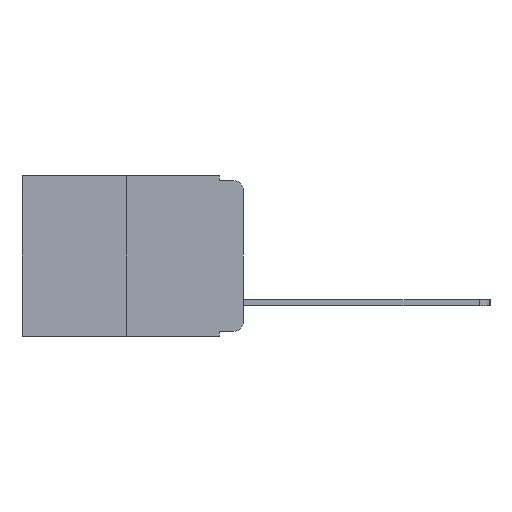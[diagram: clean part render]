
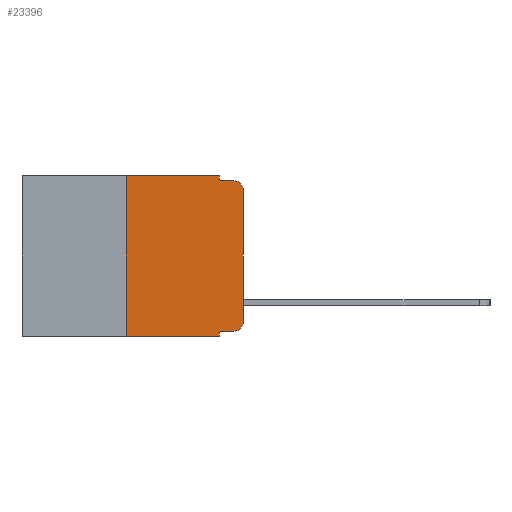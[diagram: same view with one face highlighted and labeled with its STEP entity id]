
A CAD part, left-side view. The second image highlights one B-rep face of the part: STEP entity #23396.
In plain terms, the highlighted planar face has unit normal (-1, 0, 0).
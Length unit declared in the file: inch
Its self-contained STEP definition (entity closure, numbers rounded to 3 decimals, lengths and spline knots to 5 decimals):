
#172 = LINE ( 'NONE', #19578, #9932 ) ;
#1285 = VERTEX_POINT ( 'NONE', #12604 ) ;
#1417 = ORIENTED_EDGE ( 'NONE', *, *, #24601, .T. ) ;
#1732 = CARTESIAN_POINT ( 'NONE',  ( 0., 0., -0.03 ) ) ;
#2103 = CARTESIAN_POINT ( 'NONE',  ( 0., 0.473, 0. ) ) ;
#2247 = FACE_OUTER_BOUND ( 'NONE', #20604, .T. ) ;
#2303 = CARTESIAN_POINT ( 'NONE',  ( 0., 0., 0. ) ) ;
#2648 = VERTEX_POINT ( 'NONE', #5030 ) ;
#3129 = CARTESIAN_POINT ( 'NONE',  ( 0., 0.051, -0.01 ) ) ;
#3479 = CARTESIAN_POINT ( 'NONE',  ( 0., 0.02, -0.333 ) ) ;
#3543 = ORIENTED_EDGE ( 'NONE', *, *, #11401, .T. ) ;
#3576 = VECTOR ( 'NONE', #8327, 39.37008 ) ;
#3725 = VERTEX_POINT ( 'NONE', #11868 ) ;
#3742 = EDGE_CURVE ( 'NONE', #19239, #2648, #11550, .T. ) ;
#4079 = DIRECTION ( 'NONE',  ( 0., 0., -1. ) ) ;
#4282 = DIRECTION ( 'NONE',  ( 0., 0., 1. ) ) ;
#4989 = CARTESIAN_POINT ( 'NONE',  ( 0., 0.25, 0. ) ) ;
#5030 = CARTESIAN_POINT ( 'NONE',  ( 0., 0., -0.313 ) ) ;
#5317 = VERTEX_POINT ( 'NONE', #4989 ) ;
#5421 = CARTESIAN_POINT ( 'NONE',  ( 0., 0.051, -0.01 ) ) ;
#5952 = VECTOR ( 'NONE', #24558, 39.37008 ) ;
#5959 = VECTOR ( 'NONE', #7325, 39.37008 ) ;
#6281 = CIRCLE ( 'NONE', #14288, 0.02 ) ;
#6355 = ORIENTED_EDGE ( 'NONE', *, *, #17832, .F. ) ;
#6842 = VERTEX_POINT ( 'NONE', #1732 ) ;
#7205 = EDGE_CURVE ( 'NONE', #6842, #19594, #6281, .T. ) ;
#7266 = ORIENTED_EDGE ( 'NONE', *, *, #7205, .T. ) ;
#7325 = DIRECTION ( 'NONE',  ( 0., -1., 0. ) ) ;
#7540 = VECTOR ( 'NONE', #11343, 39.37008 ) ;
#8327 = DIRECTION ( 'NONE',  ( 0., -1., 0. ) ) ;
#8449 = CARTESIAN_POINT ( 'NONE',  ( 0., 0.473, 0. ) ) ;
#8485 = ORIENTED_EDGE ( 'NONE', *, *, #20113, .F. ) ;
#8624 = CARTESIAN_POINT ( 'NONE',  ( 0., 0.02, -0.01 ) ) ;
#8637 = VECTOR ( 'NONE', #4282, 39.37008 ) ;
#9074 = ORIENTED_EDGE ( 'NONE', *, *, #22589, .F. ) ;
#9227 = LINE ( 'NONE', #2303, #8637 ) ;
#9397 = CARTESIAN_POINT ( 'NONE',  ( 0., 0.051, 0. ) ) ;
#9544 = VERTEX_POINT ( 'NONE', #23968 ) ;
#9932 = VECTOR ( 'NONE', #23350, 39.37008 ) ;
#10011 = CARTESIAN_POINT ( 'NONE',  ( 0., 0.02, -0.313 ) ) ;
#10608 = CARTESIAN_POINT ( 'NONE',  ( 0., 0.02, -0.03 ) ) ;
#11343 = DIRECTION ( 'NONE',  ( 0., 0., -1. ) ) ;
#11401 = EDGE_CURVE ( 'NONE', #13711, #19239, #13958, .T. ) ;
#11477 = ORIENTED_EDGE ( 'NONE', *, *, #22832, .F. ) ;
#11550 = CIRCLE ( 'NONE', #17213, 0.02 ) ;
#11707 = LINE ( 'NONE', #15319, #5952 ) ;
#11868 = CARTESIAN_POINT ( 'NONE',  ( 0., 0.051, 0. ) ) ;
#11964 = DIRECTION ( 'NONE',  ( 0., 0., -1. ) ) ;
#12585 = DIRECTION ( 'NONE',  ( 0., 0., -1. ) ) ;
#12604 = CARTESIAN_POINT ( 'NONE',  ( 0., 0.051, -0.343 ) ) ;
#12703 = LINE ( 'NONE', #9397, #7540 ) ;
#13164 = VECTOR ( 'NONE', #22785, 39.37008 ) ;
#13711 = VERTEX_POINT ( 'NONE', #20952 ) ;
#13756 = LINE ( 'NONE', #20962, #13164 ) ;
#13958 = LINE ( 'NONE', #16002, #3576 ) ;
#14231 = EDGE_CURVE ( 'NONE', #9544, #1285, #11707, .T. ) ;
#14288 = AXIS2_PLACEMENT_3D ( 'NONE', #10608, #23798, #12585 ) ;
#15319 = CARTESIAN_POINT ( 'NONE',  ( 0., 0.473, -0.343 ) ) ;
#15429 = ORIENTED_EDGE ( 'NONE', *, *, #21897, .F. ) ;
#15718 = DIRECTION ( 'NONE',  ( 1., 0., 0. ) ) ;
#16002 = CARTESIAN_POINT ( 'NONE',  ( 0., 0.051, -0.333 ) ) ;
#16252 = LINE ( 'NONE', #5421, #5959 ) ;
#17094 = LINE ( 'NONE', #8449, #22614 ) ;
#17213 = AXIS2_PLACEMENT_3D ( 'NONE', #10011, #23212, #11964 ) ;
#17832 = EDGE_CURVE ( 'NONE', #5317, #3725, #17094, .T. ) ;
#19239 = VERTEX_POINT ( 'NONE', #3479 ) ;
#19391 = PLANE ( 'NONE',  #20405 ) ;
#19526 = ORIENTED_EDGE ( 'NONE', *, *, #3742, .T. ) ;
#19578 = CARTESIAN_POINT ( 'NONE',  ( 0., 0.25, 0. ) ) ;
#19594 = VERTEX_POINT ( 'NONE', #8624 ) ;
#19877 = DIRECTION ( 'NONE',  ( 0., -1., 0. ) ) ;
#20113 = EDGE_CURVE ( 'NONE', #13711, #1285, #13756, .T. ) ;
#20405 = AXIS2_PLACEMENT_3D ( 'NONE', #2103, #15718, #4079 ) ;
#20602 = VERTEX_POINT ( 'NONE', #3129 ) ;
#20604 = EDGE_LOOP ( 'NONE', ( #1417, #7266, #9074, #15429, #6355, #11477, #22133, #8485, #3543, #19526 ) ) ;
#20952 = CARTESIAN_POINT ( 'NONE',  ( 0., 0.051, -0.333 ) ) ;
#20962 = CARTESIAN_POINT ( 'NONE',  ( 0., 0.051, 0. ) ) ;
#21897 = EDGE_CURVE ( 'NONE', #3725, #20602, #12703, .T. ) ;
#22133 = ORIENTED_EDGE ( 'NONE', *, *, #14231, .T. ) ;
#22589 = EDGE_CURVE ( 'NONE', #20602, #19594, #16252, .T. ) ;
#22614 = VECTOR ( 'NONE', #19877, 39.37008 ) ;
#22785 = DIRECTION ( 'NONE',  ( 0., 0., -1. ) ) ;
#22832 = EDGE_CURVE ( 'NONE', #9544, #5317, #172, .T. ) ;
#23212 = DIRECTION ( 'NONE',  ( -1., 0., 0. ) ) ;
#23350 = DIRECTION ( 'NONE',  ( 0., 0., 1. ) ) ;
#23396 = ADVANCED_FACE ( 'NONE', ( #2247 ), #19391, .F. ) ;
#23798 = DIRECTION ( 'NONE',  ( -1., 0., 0. ) ) ;
#23968 = CARTESIAN_POINT ( 'NONE',  ( 0., 0.25, -0.343 ) ) ;
#24558 = DIRECTION ( 'NONE',  ( 0., -1., 0. ) ) ;
#24601 = EDGE_CURVE ( 'NONE', #2648, #6842, #9227, .T. ) ;
